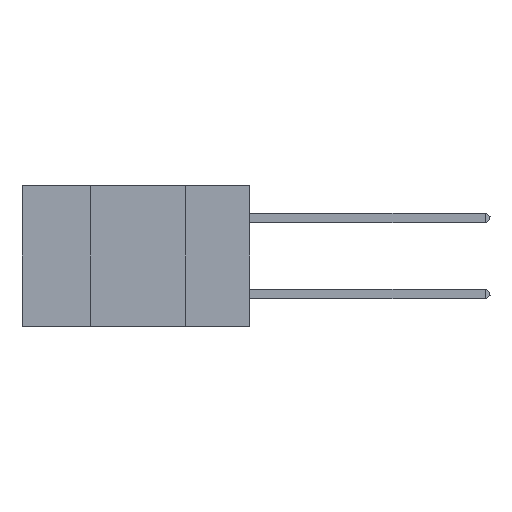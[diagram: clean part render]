
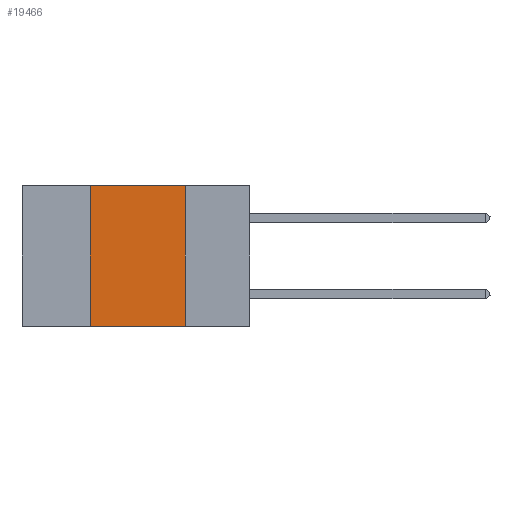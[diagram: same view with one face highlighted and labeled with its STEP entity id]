
A CAD part, left-side view. The second image highlights one B-rep face of the part: STEP entity #19466.
In plain terms, the highlighted planar face has unit normal (-1, 0, 0).
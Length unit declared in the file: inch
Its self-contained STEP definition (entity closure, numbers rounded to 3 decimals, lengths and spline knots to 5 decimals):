
#468 = CARTESIAN_POINT ( 'NONE',  ( 0., 0.6, 0. ) ) ;
#2151 = LINE ( 'NONE', #43738, #25771 ) ;
#2532 = CARTESIAN_POINT ( 'NONE',  ( 0., 0.6, -0.37 ) ) ;
#3097 = EDGE_CURVE ( 'NONE', #5659, #40425, #20603, .T. ) ;
#3867 = CARTESIAN_POINT ( 'NONE',  ( 0., 0.42, -0.37 ) ) ;
#4541 = LINE ( 'NONE', #38086, #37756 ) ;
#5659 = VERTEX_POINT ( 'NONE', #3867 ) ;
#6497 = ORIENTED_EDGE ( 'NONE', *, *, #20456, .F. ) ;
#6928 = DIRECTION ( 'NONE',  ( 0., 0., 1. ) ) ;
#7114 = EDGE_CURVE ( 'NONE', #10384, #40425, #41065, .T. ) ;
#10384 = VERTEX_POINT ( 'NONE', #29159 ) ;
#11025 = DIRECTION ( 'NONE',  ( 1., 0., 0. ) ) ;
#11067 = ORIENTED_EDGE ( 'NONE', *, *, #7114, .F. ) ;
#11072 = VECTOR ( 'NONE', #38548, 39.37008 ) ;
#11625 = ORIENTED_EDGE ( 'NONE', *, *, #45874, .F. ) ;
#13023 = EDGE_LOOP ( 'NONE', ( #11067, #6497, #11625, #31813 ) ) ;
#15930 = DIRECTION ( 'NONE',  ( 0., 0., -1. ) ) ;
#17774 = CARTESIAN_POINT ( 'NONE',  ( 0., 0.42, 0. ) ) ;
#19466 = ADVANCED_FACE ( 'NONE', ( #34931 ), #21845, .F. ) ;
#20456 = EDGE_CURVE ( 'NONE', #21409, #10384, #2151, .T. ) ;
#20603 = LINE ( 'NONE', #2532, #11072 ) ;
#21409 = VERTEX_POINT ( 'NONE', #17774 ) ;
#21845 = PLANE ( 'NONE',  #43259 ) ;
#22599 = DIRECTION ( 'NONE',  ( 0., -1., 0. ) ) ;
#25771 = VECTOR ( 'NONE', #22599, 39.37008 ) ;
#29159 = CARTESIAN_POINT ( 'NONE',  ( 0., 0.17, 0. ) ) ;
#29755 = CARTESIAN_POINT ( 'NONE',  ( 0., 0.17, 0. ) ) ;
#31813 = ORIENTED_EDGE ( 'NONE', *, *, #3097, .T. ) ;
#34931 = FACE_OUTER_BOUND ( 'NONE', #13023, .T. ) ;
#37756 = VECTOR ( 'NONE', #6928, 39.37008 ) ;
#38086 = CARTESIAN_POINT ( 'NONE',  ( 0., 0.42, 0. ) ) ;
#38548 = DIRECTION ( 'NONE',  ( 0., -1., 0. ) ) ;
#39946 = VECTOR ( 'NONE', #15930, 39.37008 ) ;
#40425 = VERTEX_POINT ( 'NONE', #42067 ) ;
#41065 = LINE ( 'NONE', #29755, #39946 ) ;
#42067 = CARTESIAN_POINT ( 'NONE',  ( 0., 0.17, -0.37 ) ) ;
#43259 = AXIS2_PLACEMENT_3D ( 'NONE', #468, #11025, #43280 ) ;
#43280 = DIRECTION ( 'NONE',  ( 0., 0., -1. ) ) ;
#43738 = CARTESIAN_POINT ( 'NONE',  ( 0., 0.6, 0. ) ) ;
#45874 = EDGE_CURVE ( 'NONE', #5659, #21409, #4541, .T. ) ;
